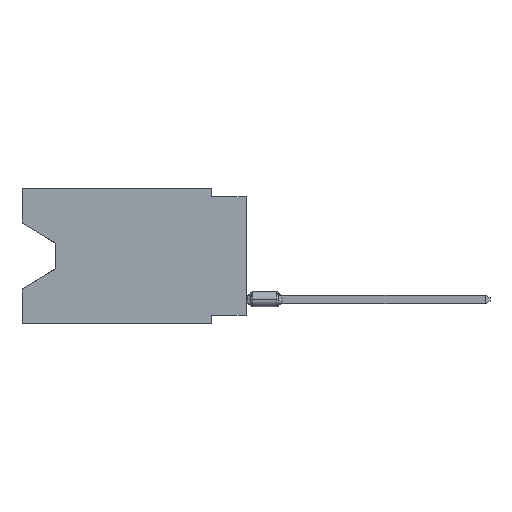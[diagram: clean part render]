
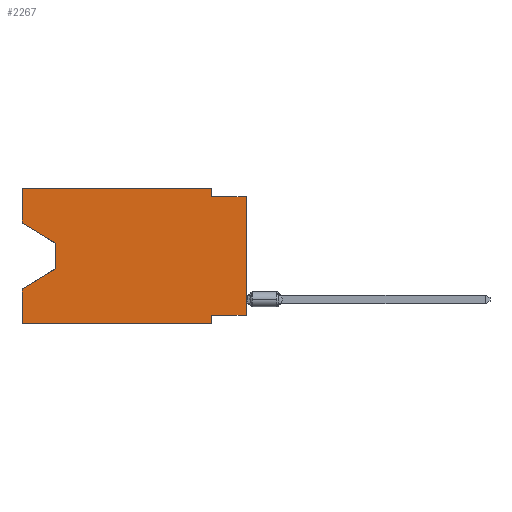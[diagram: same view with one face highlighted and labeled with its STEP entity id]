
A CAD part, left-side view. The second image highlights one B-rep face of the part: STEP entity #2267.
In plain terms, the highlighted planar face has unit normal (-1, 0, 0).
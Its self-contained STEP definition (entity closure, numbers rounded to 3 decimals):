
#13 = LINE ( 'NONE', #4473, #884 ) ;
#238 = VERTEX_POINT ( 'NONE', #10957 ) ;
#297 = LINE ( 'NONE', #2530, #13884 ) ;
#312 = VECTOR ( 'NONE', #2640, 1000. ) ;
#315 = VERTEX_POINT ( 'NONE', #2491 ) ;
#357 = EDGE_LOOP ( 'NONE', ( #8021, #3778, #4728, #1148, #2671, #9548, #10398, #10809, #12125, #13122, #10069, #12506 ) ) ;
#570 = LINE ( 'NONE', #8256, #7821 ) ;
#687 = EDGE_CURVE ( 'NONE', #2478, #6539, #297, .T. ) ;
#818 = LINE ( 'NONE', #7498, #13813 ) ;
#869 = DIRECTION ( 'NONE',  ( 0., 0., -1. ) ) ;
#884 = VECTOR ( 'NONE', #8854, 1000. ) ;
#1148 = ORIENTED_EDGE ( 'NONE', *, *, #13019, .F. ) ;
#1238 = DIRECTION ( 'NONE',  ( 0., 0., 1. ) ) ;
#1700 = EDGE_CURVE ( 'NONE', #10048, #4237, #4311, .T. ) ;
#1847 = CARTESIAN_POINT ( 'NONE',  ( 0., 2.54, -9.271 ) ) ;
#1897 = VECTOR ( 'NONE', #12211, 1000. ) ;
#1920 = EDGE_CURVE ( 'NONE', #6539, #238, #10568, .T. ) ;
#2267 = ADVANCED_FACE ( 'NONE', ( #10721 ), #6273, .F. ) ;
#2324 = DIRECTION ( 'NONE',  ( 0., -1., 0. ) ) ;
#2431 = CARTESIAN_POINT ( 'NONE',  ( 0., 2.54, -9.906 ) ) ;
#2478 = VERTEX_POINT ( 'NONE', #6667 ) ;
#2491 = CARTESIAN_POINT ( 'NONE',  ( 0., 2.54, -9.906 ) ) ;
#2530 = CARTESIAN_POINT ( 'NONE',  ( 0., 13.97, -4.013 ) ) ;
#2640 = DIRECTION ( 'NONE',  ( 0., -1., 0. ) ) ;
#2671 = ORIENTED_EDGE ( 'NONE', *, *, #12868, .T. ) ;
#2988 = VERTEX_POINT ( 'NONE', #13165 ) ;
#3010 = CARTESIAN_POINT ( 'NONE',  ( 0., 13.97, -5.893 ) ) ;
#3250 = LINE ( 'NONE', #5474, #13973 ) ;
#3338 = EDGE_CURVE ( 'NONE', #13154, #2478, #13, .T. ) ;
#3652 = EDGE_CURVE ( 'NONE', #13154, #9347, #7340, .T. ) ;
#3778 = ORIENTED_EDGE ( 'NONE', *, *, #687, .T. ) ;
#3836 = VERTEX_POINT ( 'NONE', #6903 ) ;
#4147 = VECTOR ( 'NONE', #13393, 1000. ) ;
#4167 = CARTESIAN_POINT ( 'NONE',  ( 0., 16.383, 0. ) ) ;
#4237 = VERTEX_POINT ( 'NONE', #9292 ) ;
#4311 = LINE ( 'NONE', #4460, #13238 ) ;
#4460 = CARTESIAN_POINT ( 'NONE',  ( 0., 0., -0.635 ) ) ;
#4473 = CARTESIAN_POINT ( 'NONE',  ( 0., 16.383, -2.546 ) ) ;
#4728 = ORIENTED_EDGE ( 'NONE', *, *, #1920, .T. ) ;
#5090 = VECTOR ( 'NONE', #1238, 1000. ) ;
#5187 = DIRECTION ( 'NONE',  ( 1., 0., 0. ) ) ;
#5347 = DIRECTION ( 'NONE',  ( 0., 0., 1. ) ) ;
#5474 = CARTESIAN_POINT ( 'NONE',  ( 0., 16.383, 0. ) ) ;
#5694 = DIRECTION ( 'NONE',  ( 0., -1., 0. ) ) ;
#6273 = PLANE ( 'NONE',  #8898 ) ;
#6539 = VERTEX_POINT ( 'NONE', #3010 ) ;
#6575 = EDGE_CURVE ( 'NONE', #3836, #10048, #570, .T. ) ;
#6667 = CARTESIAN_POINT ( 'NONE',  ( 0., 13.97, -4.013 ) ) ;
#6903 = CARTESIAN_POINT ( 'NONE',  ( 0., 2.54, 0. ) ) ;
#7340 = LINE ( 'NONE', #4167, #10995 ) ;
#7400 = DIRECTION ( 'NONE',  ( 0., 0.855, -0.519 ) ) ;
#7498 = CARTESIAN_POINT ( 'NONE',  ( 0., 16.383, 0. ) ) ;
#7790 = CARTESIAN_POINT ( 'NONE',  ( 0., 16.383, -2.546 ) ) ;
#7821 = VECTOR ( 'NONE', #8459, 1000. ) ;
#8021 = ORIENTED_EDGE ( 'NONE', *, *, #3338, .T. ) ;
#8234 = VERTEX_POINT ( 'NONE', #10455 ) ;
#8256 = CARTESIAN_POINT ( 'NONE',  ( 0., 2.54, 0. ) ) ;
#8351 = DIRECTION ( 'NONE',  ( 0., 0., 1. ) ) ;
#8459 = DIRECTION ( 'NONE',  ( 0., 0., -1. ) ) ;
#8777 = LINE ( 'NONE', #11089, #5090 ) ;
#8854 = DIRECTION ( 'NONE',  ( 0., -0.855, -0.519 ) ) ;
#8898 = AXIS2_PLACEMENT_3D ( 'NONE', #9713, #5187, #869 ) ;
#9250 = LINE ( 'NONE', #9318, #312 ) ;
#9292 = CARTESIAN_POINT ( 'NONE',  ( 0., 0., -0.635 ) ) ;
#9318 = CARTESIAN_POINT ( 'NONE',  ( 0., 16.383, -9.906 ) ) ;
#9347 = VERTEX_POINT ( 'NONE', #10097 ) ;
#9548 = ORIENTED_EDGE ( 'NONE', *, *, #10733, .F. ) ;
#9713 = CARTESIAN_POINT ( 'NONE',  ( 0., 16.383, 0. ) ) ;
#9835 = EDGE_CURVE ( 'NONE', #9347, #3836, #3250, .T. ) ;
#10048 = VERTEX_POINT ( 'NONE', #11704 ) ;
#10069 = ORIENTED_EDGE ( 'NONE', *, *, #9835, .F. ) ;
#10097 = CARTESIAN_POINT ( 'NONE',  ( 0., 16.383, 0. ) ) ;
#10398 = ORIENTED_EDGE ( 'NONE', *, *, #12341, .F. ) ;
#10455 = CARTESIAN_POINT ( 'NONE',  ( 0., 16.383, -9.906 ) ) ;
#10568 = LINE ( 'NONE', #12773, #12564 ) ;
#10721 = FACE_OUTER_BOUND ( 'NONE', #357, .T. ) ;
#10733 = EDGE_CURVE ( 'NONE', #12531, #315, #12394, .T. ) ;
#10809 = ORIENTED_EDGE ( 'NONE', *, *, #11030, .T. ) ;
#10957 = CARTESIAN_POINT ( 'NONE',  ( 0., 16.383, -7.36 ) ) ;
#10995 = VECTOR ( 'NONE', #8351, 1000. ) ;
#11030 = EDGE_CURVE ( 'NONE', #2988, #4237, #8777, .T. ) ;
#11089 = CARTESIAN_POINT ( 'NONE',  ( 0., 0., 0. ) ) ;
#11427 = DIRECTION ( 'NONE',  ( 0., 0., -1. ) ) ;
#11704 = CARTESIAN_POINT ( 'NONE',  ( 0., 2.54, -0.635 ) ) ;
#12061 = CARTESIAN_POINT ( 'NONE',  ( 0., 0., -9.271 ) ) ;
#12125 = ORIENTED_EDGE ( 'NONE', *, *, #1700, .F. ) ;
#12211 = DIRECTION ( 'NONE',  ( 0., 1., 0. ) ) ;
#12341 = EDGE_CURVE ( 'NONE', #2988, #12531, #13055, .T. ) ;
#12394 = LINE ( 'NONE', #2431, #4147 ) ;
#12506 = ORIENTED_EDGE ( 'NONE', *, *, #3652, .F. ) ;
#12531 = VERTEX_POINT ( 'NONE', #1847 ) ;
#12564 = VECTOR ( 'NONE', #7400, 1000. ) ;
#12773 = CARTESIAN_POINT ( 'NONE',  ( 0., 13.97, -5.893 ) ) ;
#12868 = EDGE_CURVE ( 'NONE', #8234, #315, #9250, .T. ) ;
#13019 = EDGE_CURVE ( 'NONE', #8234, #238, #818, .T. ) ;
#13055 = LINE ( 'NONE', #12061, #1897 ) ;
#13122 = ORIENTED_EDGE ( 'NONE', *, *, #6575, .F. ) ;
#13154 = VERTEX_POINT ( 'NONE', #7790 ) ;
#13165 = CARTESIAN_POINT ( 'NONE',  ( 0., 0., -9.271 ) ) ;
#13238 = VECTOR ( 'NONE', #5694, 1000. ) ;
#13393 = DIRECTION ( 'NONE',  ( 0., 0., -1. ) ) ;
#13813 = VECTOR ( 'NONE', #5347, 1000. ) ;
#13884 = VECTOR ( 'NONE', #11427, 1000. ) ;
#13973 = VECTOR ( 'NONE', #2324, 1000. ) ;
